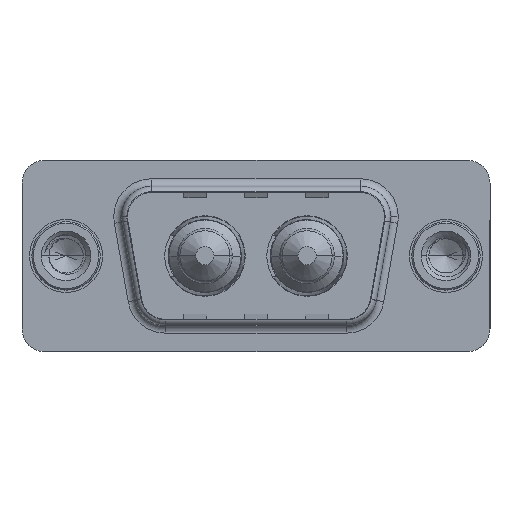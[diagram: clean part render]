
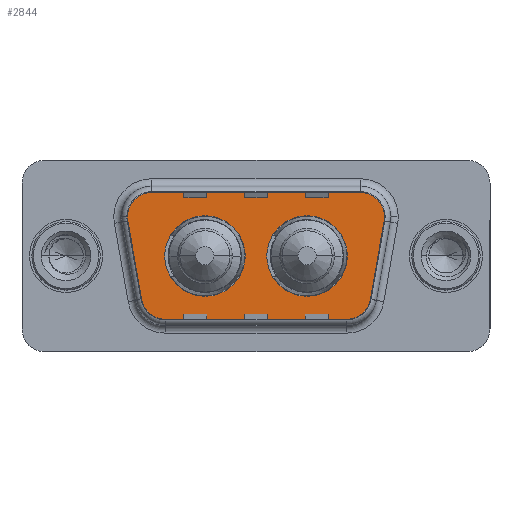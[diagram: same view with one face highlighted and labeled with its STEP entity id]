
A CAD part, top view. The second image highlights one B-rep face of the part: STEP entity #2844.
In plain terms, the highlighted planar face has unit normal (0, 0, 1).
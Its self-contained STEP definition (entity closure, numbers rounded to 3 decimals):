
#85 = VECTOR ( 'NONE', #10339, 1000. ) ;
#193 = AXIS2_PLACEMENT_3D ( 'NONE', #2524, #14154, #10115 ) ;
#227 = CARTESIAN_POINT ( 'NONE',  ( 21.534, 2.553, 0. ) ) ;
#301 = VERTEX_POINT ( 'NONE', #18485 ) ;
#396 = VECTOR ( 'NONE', #605, 1000. ) ;
#479 = AXIS2_PLACEMENT_3D ( 'NONE', #16245, #7681, #17681 ) ;
#605 = DIRECTION ( 'NONE',  ( 1., 0., 0. ) ) ;
#861 = CARTESIAN_POINT ( 'NONE',  ( 5.436, 2.9, 0. ) ) ;
#986 = VERTEX_POINT ( 'NONE', #16680 ) ;
#987 = CARTESIAN_POINT ( 'NONE',  ( 6.459, -2.9, 0. ) ) ;
#1158 = DIRECTION ( 'NONE',  ( 0., 0., 1. ) ) ;
#1293 = ORIENTED_EDGE ( 'NONE', *, *, #16717, .F. ) ;
#1492 = CARTESIAN_POINT ( 'NONE',  ( 3.466, 2.553, 0. ) ) ;
#1690 = VERTEX_POINT ( 'NONE', #13664 ) ;
#1717 = CIRCLE ( 'NONE', #11909, 2.65 ) ;
#1799 = FACE_BOUND ( 'NONE', #9075, .T. ) ;
#2198 = EDGE_CURVE ( 'NONE', #11135, #13242, #4743, .T. ) ;
#2273 = DIRECTION ( 'NONE',  ( 1., 0., 0. ) ) ;
#2280 = CARTESIAN_POINT ( 'NONE',  ( 19.564, 2.9, 0. ) ) ;
#2524 = CARTESIAN_POINT ( 'NONE',  ( 18.541, -2.9, 0. ) ) ;
#2844 = ADVANCED_FACE ( 'NONE', ( #16671, #1799, #12838 ), #9441, .T. ) ;
#2879 = DIRECTION ( 'NONE',  ( 0.174, -0.985, 0. ) ) ;
#2972 = VERTEX_POINT ( 'NONE', #13471 ) ;
#3113 = AXIS2_PLACEMENT_3D ( 'NONE', #3203, #13280, #4636 ) ;
#3179 = CIRCLE ( 'NONE', #9324, 2.65 ) ;
#3203 = CARTESIAN_POINT ( 'NONE',  ( 9.14, 0., 0. ) ) ;
#3252 = ORIENTED_EDGE ( 'NONE', *, *, #14983, .T. ) ;
#3372 = CARTESIAN_POINT ( 'NONE',  ( 18.51, 0., 0. ) ) ;
#3518 = ORIENTED_EDGE ( 'NONE', *, *, #7260, .F. ) ;
#3594 = AXIS2_PLACEMENT_3D ( 'NONE', #6223, #16253, #7698 ) ;
#3762 = DIRECTION ( 'NONE',  ( -1., 0., 0. ) ) ;
#4084 = VERTEX_POINT ( 'NONE', #12081 ) ;
#4155 = AXIS2_PLACEMENT_3D ( 'NONE', #987, #13433, #7862 ) ;
#4203 = LINE ( 'NONE', #9269, #396 ) ;
#4242 = CARTESIAN_POINT ( 'NONE',  ( 9.14, 0., 0. ) ) ;
#4419 = VERTEX_POINT ( 'NONE', #16480 ) ;
#4485 = VERTEX_POINT ( 'NONE', #12182 ) ;
#4601 = ORIENTED_EDGE ( 'NONE', *, *, #7987, .T. ) ;
#4636 = DIRECTION ( 'NONE',  ( 1., 0., 0. ) ) ;
#4743 = CIRCLE ( 'NONE', #4155, 2. ) ;
#5030 = EDGE_CURVE ( 'NONE', #1690, #986, #15398, .T. ) ;
#5186 = CIRCLE ( 'NONE', #479, 2. ) ;
#5356 = VERTEX_POINT ( 'NONE', #11077 ) ;
#5449 = EDGE_CURVE ( 'NONE', #2972, #1690, #10478, .T. ) ;
#5620 = ORIENTED_EDGE ( 'NONE', *, *, #15788, .T. ) ;
#5700 = DIRECTION ( 'NONE',  ( 1., 0., 0. ) ) ;
#5992 = ORIENTED_EDGE ( 'NONE', *, *, #13759, .T. ) ;
#6223 = CARTESIAN_POINT ( 'NONE',  ( 15.86, 0., 0. ) ) ;
#6548 = EDGE_LOOP ( 'NONE', ( #1293, #17038 ) ) ;
#6744 = CARTESIAN_POINT ( 'NONE',  ( 15.86, 0., 0. ) ) ;
#7216 = ORIENTED_EDGE ( 'NONE', *, *, #5030, .T. ) ;
#7260 = EDGE_CURVE ( 'NONE', #14145, #5356, #3179, .T. ) ;
#7530 = CARTESIAN_POINT ( 'NONE',  ( 21.564, 2.9, 0. ) ) ;
#7681 = DIRECTION ( 'NONE',  ( 0., 0., 1. ) ) ;
#7698 = DIRECTION ( 'NONE',  ( 1., 0., 0. ) ) ;
#7862 = DIRECTION ( 'NONE',  ( -1., 0., 0. ) ) ;
#7987 = EDGE_CURVE ( 'NONE', #14741, #4485, #5186, .T. ) ;
#8219 = DIRECTION ( 'NONE',  ( 1., 0., 0. ) ) ;
#8432 = DIRECTION ( 'NONE',  ( -1., 0., 0. ) ) ;
#9075 = EDGE_LOOP ( 'NONE', ( #16806, #3518 ) ) ;
#9269 = CARTESIAN_POINT ( 'NONE',  ( 6.459, -4.9, 0. ) ) ;
#9324 = AXIS2_PLACEMENT_3D ( 'NONE', #4242, #14299, #5700 ) ;
#9441 = PLANE ( 'NONE',  #193 ) ;
#9800 = EDGE_CURVE ( 'NONE', #13242, #2972, #4203, .T. ) ;
#9808 = CARTESIAN_POINT ( 'NONE',  ( 18.541, -2.9, 0. ) ) ;
#10115 = DIRECTION ( 'NONE',  ( 1., 0., 0. ) ) ;
#10324 = CARTESIAN_POINT ( 'NONE',  ( 6.459, -4.9, 0. ) ) ;
#10339 = DIRECTION ( 'NONE',  ( 0.174, 0.985, 0. ) ) ;
#10437 = ORIENTED_EDGE ( 'NONE', *, *, #5449, .T. ) ;
#10478 = CIRCLE ( 'NONE', #18486, 2. ) ;
#10756 = CIRCLE ( 'NONE', #12978, 2. ) ;
#10868 = CARTESIAN_POINT ( 'NONE',  ( 4.489, -3.247, 0. ) ) ;
#10973 = DIRECTION ( 'NONE',  ( 0., 0., 1. ) ) ;
#11039 = CARTESIAN_POINT ( 'NONE',  ( 6.49, 0., 0. ) ) ;
#11077 = CARTESIAN_POINT ( 'NONE',  ( 11.79, 0., 0. ) ) ;
#11135 = VERTEX_POINT ( 'NONE', #10868 ) ;
#11258 = DIRECTION ( 'NONE',  ( 1., 0., 0. ) ) ;
#11909 = AXIS2_PLACEMENT_3D ( 'NONE', #6744, #16757, #8219 ) ;
#12081 = CARTESIAN_POINT ( 'NONE',  ( 3.466, 2.553, 0. ) ) ;
#12115 = ORIENTED_EDGE ( 'NONE', *, *, #9800, .T. ) ;
#12182 = CARTESIAN_POINT ( 'NONE',  ( 19.564, 4.9, 0. ) ) ;
#12391 = DIRECTION ( 'NONE',  ( 0., 0., 1. ) ) ;
#12696 = VERTEX_POINT ( 'NONE', #3372 ) ;
#12838 = FACE_OUTER_BOUND ( 'NONE', #12977, .T. ) ;
#12977 = EDGE_LOOP ( 'NONE', ( #10437, #7216, #3252, #4601, #5620, #16443, #5992, #15044, #12115 ) ) ;
#12978 = AXIS2_PLACEMENT_3D ( 'NONE', #861, #10973, #2273 ) ;
#13197 = LINE ( 'NONE', #15521, #16998 ) ;
#13242 = VERTEX_POINT ( 'NONE', #10324 ) ;
#13280 = DIRECTION ( 'NONE',  ( 0., 0., 1. ) ) ;
#13433 = DIRECTION ( 'NONE',  ( 0., 0., 1. ) ) ;
#13471 = CARTESIAN_POINT ( 'NONE',  ( 18.541, -4.9, 0. ) ) ;
#13664 = CARTESIAN_POINT ( 'NONE',  ( 20.511, -3.247, 0. ) ) ;
#13666 = CIRCLE ( 'NONE', #18589, 2. ) ;
#13759 = EDGE_CURVE ( 'NONE', #4084, #11135, #14132, .T. ) ;
#14132 = LINE ( 'NONE', #1492, #16614 ) ;
#14145 = VERTEX_POINT ( 'NONE', #11039 ) ;
#14154 = DIRECTION ( 'NONE',  ( 0., 0., 1. ) ) ;
#14299 = DIRECTION ( 'NONE',  ( 0., 0., 1. ) ) ;
#14741 = VERTEX_POINT ( 'NONE', #7530 ) ;
#14983 = EDGE_CURVE ( 'NONE', #986, #14741, #13666, .T. ) ;
#15044 = ORIENTED_EDGE ( 'NONE', *, *, #2198, .T. ) ;
#15072 = EDGE_CURVE ( 'NONE', #4419, #12696, #1717, .T. ) ;
#15169 = CIRCLE ( 'NONE', #3113, 2.65 ) ;
#15398 = LINE ( 'NONE', #227, #85 ) ;
#15521 = CARTESIAN_POINT ( 'NONE',  ( 5.436, 4.9, 0. ) ) ;
#15788 = EDGE_CURVE ( 'NONE', #4485, #301, #13197, .T. ) ;
#16245 = CARTESIAN_POINT ( 'NONE',  ( 19.564, 2.9, 0. ) ) ;
#16253 = DIRECTION ( 'NONE',  ( 0., 0., 1. ) ) ;
#16382 = EDGE_CURVE ( 'NONE', #301, #4084, #10756, .T. ) ;
#16443 = ORIENTED_EDGE ( 'NONE', *, *, #16382, .T. ) ;
#16480 = CARTESIAN_POINT ( 'NONE',  ( 13.21, 0., 0. ) ) ;
#16614 = VECTOR ( 'NONE', #2879, 1000. ) ;
#16671 = FACE_BOUND ( 'NONE', #6548, .T. ) ;
#16680 = CARTESIAN_POINT ( 'NONE',  ( 21.534, 2.553, 0. ) ) ;
#16717 = EDGE_CURVE ( 'NONE', #12696, #4419, #18535, .T. ) ;
#16757 = DIRECTION ( 'NONE',  ( 0., 0., 1. ) ) ;
#16806 = ORIENTED_EDGE ( 'NONE', *, *, #18042, .F. ) ;
#16998 = VECTOR ( 'NONE', #8432, 1000. ) ;
#17038 = ORIENTED_EDGE ( 'NONE', *, *, #15072, .F. ) ;
#17681 = DIRECTION ( 'NONE',  ( -1., 0., 0. ) ) ;
#18042 = EDGE_CURVE ( 'NONE', #5356, #14145, #15169, .T. ) ;
#18485 = CARTESIAN_POINT ( 'NONE',  ( 5.436, 4.9, 0. ) ) ;
#18486 = AXIS2_PLACEMENT_3D ( 'NONE', #9808, #1158, #11258 ) ;
#18535 = CIRCLE ( 'NONE', #3594, 2.65 ) ;
#18589 = AXIS2_PLACEMENT_3D ( 'NONE', #2280, #12391, #3762 ) ;
